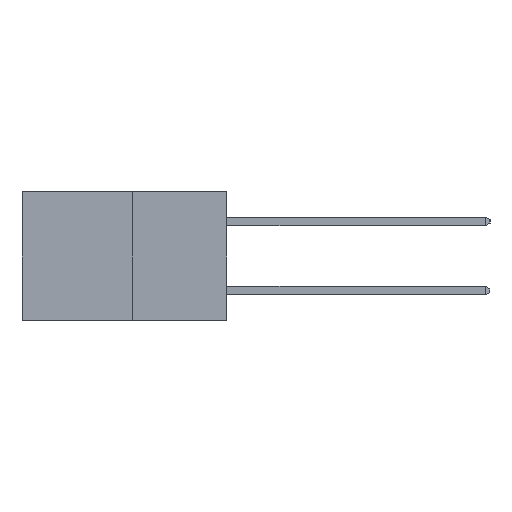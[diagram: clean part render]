
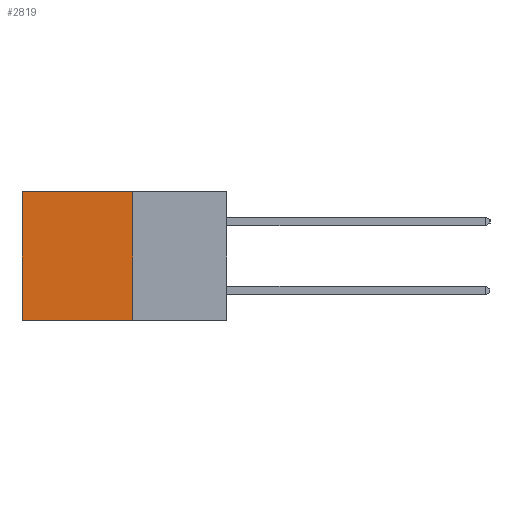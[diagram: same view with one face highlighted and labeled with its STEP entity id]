
A CAD part, left-side view. The second image highlights one B-rep face of the part: STEP entity #2819.
In plain terms, the highlighted planar face has unit normal (-1, 0, 0).
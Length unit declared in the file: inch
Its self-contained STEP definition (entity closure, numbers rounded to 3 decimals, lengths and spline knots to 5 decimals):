
#83 = CARTESIAN_POINT ( 'NONE',  ( 0.277, 0.59, 0. ) ) ;
#1437 = DIRECTION ( 'NONE',  ( 1., 0., 0. ) ) ;
#1739 = EDGE_CURVE ( 'NONE', #9163, #11312, #3494, .T. ) ;
#2808 = LINE ( 'NONE', #18511, #15179 ) ;
#2819 = ADVANCED_FACE ( 'NONE', ( #16504 ), #3398, .F. ) ;
#3161 = CARTESIAN_POINT ( 'NONE',  ( 0.277, 0.27, -0.37 ) ) ;
#3398 = PLANE ( 'NONE',  #5181 ) ;
#3494 = LINE ( 'NONE', #19138, #15333 ) ;
#3914 = DIRECTION ( 'NONE',  ( 0., 0., -1. ) ) ;
#5003 = DIRECTION ( 'NONE',  ( 0., 0., -1. ) ) ;
#5181 = AXIS2_PLACEMENT_3D ( 'NONE', #3161, #1437, #3914 ) ;
#5264 = VECTOR ( 'NONE', #20567, 39.37008 ) ;
#6736 = EDGE_LOOP ( 'NONE', ( #18901, #11566, #15757, #7793 ) ) ;
#7793 = ORIENTED_EDGE ( 'NONE', *, *, #1739, .T. ) ;
#8555 = VERTEX_POINT ( 'NONE', #13509 ) ;
#8690 = VECTOR ( 'NONE', #5003, 39.37008 ) ;
#9163 = VERTEX_POINT ( 'NONE', #16071 ) ;
#11312 = VERTEX_POINT ( 'NONE', #83 ) ;
#11444 = CARTESIAN_POINT ( 'NONE',  ( 0.277, 0.27, -0.37 ) ) ;
#11566 = ORIENTED_EDGE ( 'NONE', *, *, #16364, .F. ) ;
#13509 = CARTESIAN_POINT ( 'NONE',  ( 0.277, 0.27, -0.37 ) ) ;
#13836 = LINE ( 'NONE', #19057, #5264 ) ;
#14366 = CARTESIAN_POINT ( 'NONE',  ( 0.277, 0.59, -0.37 ) ) ;
#14461 = LINE ( 'NONE', #11444, #8690 ) ;
#14914 = EDGE_CURVE ( 'NONE', #11312, #15143, #2808, .T. ) ;
#15143 = VERTEX_POINT ( 'NONE', #14366 ) ;
#15179 = VECTOR ( 'NONE', #20044, 39.37008 ) ;
#15333 = VECTOR ( 'NONE', #18761, 39.37008 ) ;
#15757 = ORIENTED_EDGE ( 'NONE', *, *, #19029, .F. ) ;
#16071 = CARTESIAN_POINT ( 'NONE',  ( 0.277, 0.27, 0. ) ) ;
#16364 = EDGE_CURVE ( 'NONE', #8555, #15143, #13836, .T. ) ;
#16504 = FACE_OUTER_BOUND ( 'NONE', #6736, .T. ) ;
#18511 = CARTESIAN_POINT ( 'NONE',  ( 0.277, 0.59, -0.37 ) ) ;
#18761 = DIRECTION ( 'NONE',  ( 0., 1., 0. ) ) ;
#18901 = ORIENTED_EDGE ( 'NONE', *, *, #14914, .T. ) ;
#19029 = EDGE_CURVE ( 'NONE', #9163, #8555, #14461, .T. ) ;
#19057 = CARTESIAN_POINT ( 'NONE',  ( 0.277, 0.27, -0.37 ) ) ;
#19138 = CARTESIAN_POINT ( 'NONE',  ( 0.277, 0.27, 0. ) ) ;
#20044 = DIRECTION ( 'NONE',  ( 0., 0., -1. ) ) ;
#20567 = DIRECTION ( 'NONE',  ( 0., 1., 0. ) ) ;
